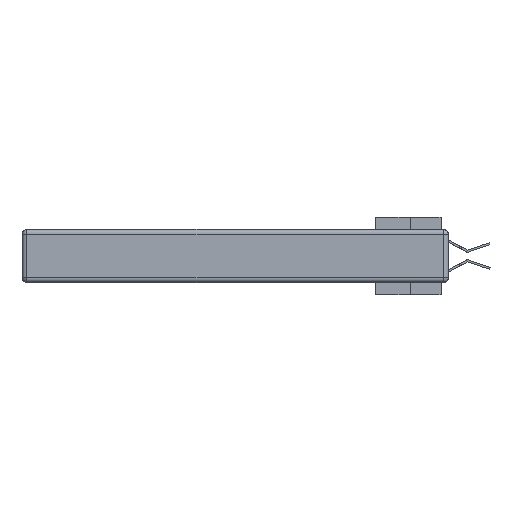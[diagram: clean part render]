
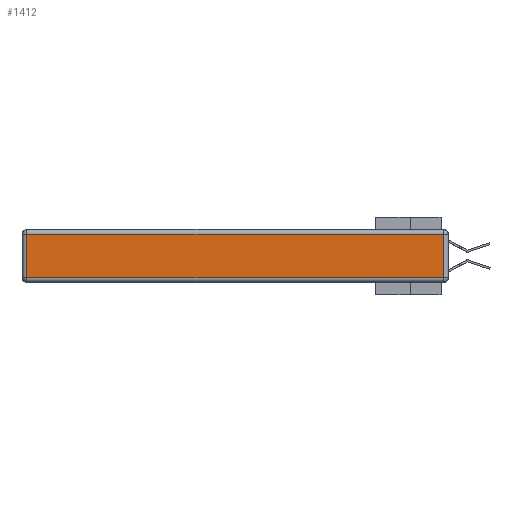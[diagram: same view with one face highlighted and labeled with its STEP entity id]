
A CAD part, left-side view. The second image highlights one B-rep face of the part: STEP entity #1412.
In plain terms, the highlighted planar face has unit normal (-1, 0, 0).
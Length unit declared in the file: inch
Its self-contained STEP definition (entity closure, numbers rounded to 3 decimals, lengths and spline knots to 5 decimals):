
#945 = VECTOR ( 'NONE', #3593, 39.37008 ) ;
#1412 = ADVANCED_FACE ( 'NONE', ( #9066 ), #18791, .T. ) ;
#3272 = VECTOR ( 'NONE', #6316, 39.37008 ) ;
#3593 = DIRECTION ( 'NONE',  ( 0., -1., 0. ) ) ;
#5068 = CARTESIAN_POINT ( 'NONE',  ( 0., 2.75, -0.03 ) ) ;
#6101 = VECTOR ( 'NONE', #28549, 39.37008 ) ;
#6316 = DIRECTION ( 'NONE',  ( 0., 0., -1. ) ) ;
#6669 = DIRECTION ( 'NONE',  ( 0., 0., 1. ) ) ;
#7348 = VERTEX_POINT ( 'NONE', #30317 ) ;
#8102 = ORIENTED_EDGE ( 'NONE', *, *, #16073, .T. ) ;
#8716 = LINE ( 'NONE', #28144, #3272 ) ;
#9066 = FACE_OUTER_BOUND ( 'NONE', #9439, .T. ) ;
#9229 = LINE ( 'NONE', #31194, #24576 ) ;
#9302 = CARTESIAN_POINT ( 'NONE',  ( 0., 0.03, -0.313 ) ) ;
#9439 = EDGE_LOOP ( 'NONE', ( #8102, #29566, #29693, #19057 ) ) ;
#12717 = CARTESIAN_POINT ( 'NONE',  ( 0., 0., -0.313 ) ) ;
#15486 = VERTEX_POINT ( 'NONE', #9302 ) ;
#16073 = EDGE_CURVE ( 'NONE', #28518, #15486, #29584, .T. ) ;
#17329 = EDGE_CURVE ( 'NONE', #20172, #7348, #26911, .T. ) ;
#18791 = PLANE ( 'NONE',  #30570 ) ;
#18945 = DIRECTION ( 'NONE',  ( 0., 0., 1. ) ) ;
#19057 = ORIENTED_EDGE ( 'NONE', *, *, #28785, .T. ) ;
#20172 = VERTEX_POINT ( 'NONE', #25197 ) ;
#20196 = CARTESIAN_POINT ( 'NONE',  ( 0., 2.72, -0.313 ) ) ;
#24576 = VECTOR ( 'NONE', #18945, 39.37008 ) ;
#25197 = CARTESIAN_POINT ( 'NONE',  ( 0., 0.03, -0.03 ) ) ;
#26115 = DIRECTION ( 'NONE',  ( -1., 0., 0. ) ) ;
#26911 = LINE ( 'NONE', #5068, #6101 ) ;
#27143 = EDGE_CURVE ( 'NONE', #15486, #20172, #9229, .T. ) ;
#28144 = CARTESIAN_POINT ( 'NONE',  ( 0., 2.72, -0.343 ) ) ;
#28518 = VERTEX_POINT ( 'NONE', #20196 ) ;
#28549 = DIRECTION ( 'NONE',  ( 0., 1., 0. ) ) ;
#28785 = EDGE_CURVE ( 'NONE', #7348, #28518, #8716, .T. ) ;
#29566 = ORIENTED_EDGE ( 'NONE', *, *, #27143, .T. ) ;
#29584 = LINE ( 'NONE', #12717, #945 ) ;
#29693 = ORIENTED_EDGE ( 'NONE', *, *, #17329, .T. ) ;
#30317 = CARTESIAN_POINT ( 'NONE',  ( 0., 2.72, -0.03 ) ) ;
#30570 = AXIS2_PLACEMENT_3D ( 'NONE', #30718, #26115, #6669 ) ;
#30718 = CARTESIAN_POINT ( 'NONE',  ( 0., 0., -0.343 ) ) ;
#31194 = CARTESIAN_POINT ( 'NONE',  ( 0., 0.03, -0.343 ) ) ;
